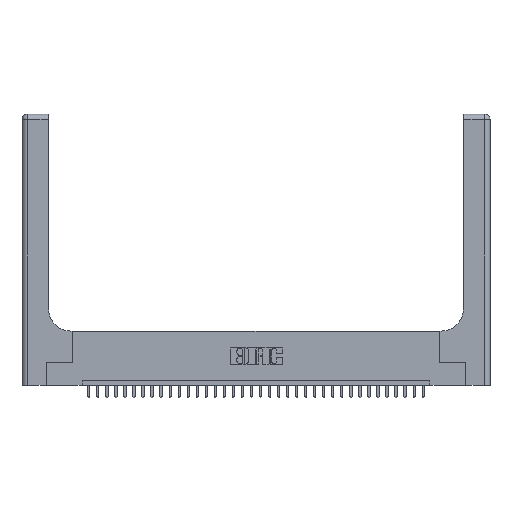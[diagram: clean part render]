
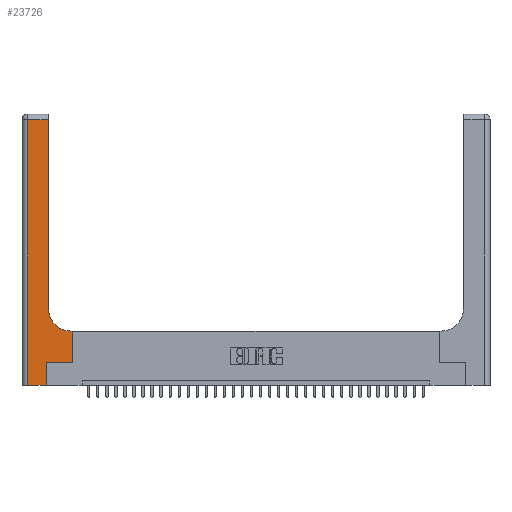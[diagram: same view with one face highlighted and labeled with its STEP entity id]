
A CAD part, top view. The second image highlights one B-rep face of the part: STEP entity #23726.
In plain terms, the highlighted planar face has unit normal (0, 0, 1).
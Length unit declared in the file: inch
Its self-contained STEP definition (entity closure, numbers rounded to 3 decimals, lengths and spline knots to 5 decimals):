
#28 = AXIS2_PLACEMENT_3D ( 'NONE', #9016, #14420, #17195 ) ;
#108 = CARTESIAN_POINT ( 'NONE',  ( 0.06, 0., 0.37 ) ) ;
#949 = VERTEX_POINT ( 'NONE', #8514 ) ;
#1142 = VERTEX_POINT ( 'NONE', #10411 ) ;
#1593 = EDGE_CURVE ( 'NONE', #949, #24150, #19657, .T. ) ;
#1617 = DIRECTION ( 'NONE',  ( 0., -1., 0. ) ) ;
#1848 = DIRECTION ( 'NONE',  ( 1., 0., 0. ) ) ;
#2084 = CARTESIAN_POINT ( 'NONE',  ( 0.269, 0.25, 0.37 ) ) ;
#3332 = CARTESIAN_POINT ( 'NONE',  ( 0.5415, 0.6, 0.37 ) ) ;
#3934 = LINE ( 'NONE', #2084, #21708 ) ;
#3965 = DIRECTION ( 'NONE',  ( -1., 0., 0. ) ) ;
#4479 = VERTEX_POINT ( 'NONE', #31100 ) ;
#5057 = DIRECTION ( 'NONE',  ( -1., 0., 0. ) ) ;
#6940 = DIRECTION ( 'NONE',  ( 0., 1., 0. ) ) ;
#7277 = EDGE_CURVE ( 'NONE', #1142, #15568, #17234, .T. ) ;
#7863 = VERTEX_POINT ( 'NONE', #3332 ) ;
#8049 = ORIENTED_EDGE ( 'NONE', *, *, #18029, .T. ) ;
#8156 = VECTOR ( 'NONE', #6940, 39.37008 ) ;
#8331 = VECTOR ( 'NONE', #9552, 39.37008 ) ;
#8478 = CARTESIAN_POINT ( 'NONE',  ( 0., 2.94, 0.37 ) ) ;
#8514 = CARTESIAN_POINT ( 'NONE',  ( 0.06, 2.94, 0.37 ) ) ;
#9016 = CARTESIAN_POINT ( 'NONE',  ( 0.5415, 0.85, 0.37 ) ) ;
#9070 = VECTOR ( 'NONE', #29698, 39.37008 ) ;
#9345 = ORIENTED_EDGE ( 'NONE', *, *, #1593, .T. ) ;
#9371 = LINE ( 'NONE', #12510, #17203 ) ;
#9552 = DIRECTION ( 'NONE',  ( 1., 0., 0. ) ) ;
#9808 = ORIENTED_EDGE ( 'NONE', *, *, #16671, .T. ) ;
#10411 = CARTESIAN_POINT ( 'NONE',  ( 0.5585, 0.25, 0.37 ) ) ;
#10804 = ORIENTED_EDGE ( 'NONE', *, *, #7277, .T. ) ;
#11607 = CARTESIAN_POINT ( 'NONE',  ( 0., 3., 0.37 ) ) ;
#11647 = LINE ( 'NONE', #25682, #8331 ) ;
#12274 = CARTESIAN_POINT ( 'NONE',  ( 0.2915, 3., 0.37 ) ) ;
#12510 = CARTESIAN_POINT ( 'NONE',  ( 0.269, 0., 0.37 ) ) ;
#12980 = CARTESIAN_POINT ( 'NONE',  ( 0.2915, 2.94, 0.37 ) ) ;
#14412 = CIRCLE ( 'NONE', #28, 0.25 ) ;
#14420 = DIRECTION ( 'NONE',  ( 0., 0., -1. ) ) ;
#14799 = EDGE_CURVE ( 'NONE', #7863, #29219, #14412, .T. ) ;
#15288 = DIRECTION ( 'NONE',  ( 0., 1., 0. ) ) ;
#15568 = VERTEX_POINT ( 'NONE', #27594 ) ;
#15746 = DIRECTION ( 'NONE',  ( 0., 1., 0. ) ) ;
#15873 = EDGE_CURVE ( 'NONE', #4479, #26837, #9371, .T. ) ;
#16080 = LINE ( 'NONE', #31485, #26107 ) ;
#16084 = LINE ( 'NONE', #8478, #9070 ) ;
#16671 = EDGE_CURVE ( 'NONE', #15568, #7863, #16080, .T. ) ;
#17195 = DIRECTION ( 'NONE',  ( 1., 0., 0. ) ) ;
#17203 = VECTOR ( 'NONE', #15288, 39.37008 ) ;
#17234 = LINE ( 'NONE', #32418, #8156 ) ;
#17813 = LINE ( 'NONE', #12274, #29883 ) ;
#18029 = EDGE_CURVE ( 'NONE', #29219, #22592, #17813, .T. ) ;
#18394 = FACE_OUTER_BOUND ( 'NONE', #28026, .T. ) ;
#18837 = VECTOR ( 'NONE', #1617, 39.37008 ) ;
#19054 = ORIENTED_EDGE ( 'NONE', *, *, #15873, .T. ) ;
#19657 = LINE ( 'NONE', #22809, #18837 ) ;
#20037 = DIRECTION ( 'NONE',  ( 0., 0., -1. ) ) ;
#21046 = ORIENTED_EDGE ( 'NONE', *, *, #23815, .T. ) ;
#21708 = VECTOR ( 'NONE', #1848, 39.37008 ) ;
#22373 = ORIENTED_EDGE ( 'NONE', *, *, #14799, .T. ) ;
#22453 = EDGE_CURVE ( 'NONE', #24150, #4479, #11647, .T. ) ;
#22592 = VERTEX_POINT ( 'NONE', #12980 ) ;
#22701 = PLANE ( 'NONE',  #33259 ) ;
#22809 = CARTESIAN_POINT ( 'NONE',  ( 0.06, 3., 0.37 ) ) ;
#23487 = ORIENTED_EDGE ( 'NONE', *, *, #22453, .T. ) ;
#23726 = ADVANCED_FACE ( 'NONE', ( #18394 ), #22701, .F. ) ;
#23815 = EDGE_CURVE ( 'NONE', #26837, #1142, #3934, .T. ) ;
#24150 = VERTEX_POINT ( 'NONE', #108 ) ;
#25627 = ORIENTED_EDGE ( 'NONE', *, *, #27071, .T. ) ;
#25682 = CARTESIAN_POINT ( 'NONE',  ( 0., 0., 0.37 ) ) ;
#26107 = VECTOR ( 'NONE', #5057, 39.37008 ) ;
#26837 = VERTEX_POINT ( 'NONE', #34325 ) ;
#27071 = EDGE_CURVE ( 'NONE', #22592, #949, #16084, .T. ) ;
#27594 = CARTESIAN_POINT ( 'NONE',  ( 0.5585, 0.6, 0.37 ) ) ;
#28026 = EDGE_LOOP ( 'NONE', ( #8049, #25627, #9345, #23487, #19054, #21046, #10804, #9808, #22373 ) ) ;
#29219 = VERTEX_POINT ( 'NONE', #29317 ) ;
#29317 = CARTESIAN_POINT ( 'NONE',  ( 0.2915, 0.85, 0.37 ) ) ;
#29698 = DIRECTION ( 'NONE',  ( -1., 0., 0. ) ) ;
#29883 = VECTOR ( 'NONE', #15746, 39.37008 ) ;
#31100 = CARTESIAN_POINT ( 'NONE',  ( 0.269, 0., 0.37 ) ) ;
#31485 = CARTESIAN_POINT ( 'NONE',  ( 0.2915, 0.6, 0.37 ) ) ;
#32418 = CARTESIAN_POINT ( 'NONE',  ( 0.5585, 0.25, 0.37 ) ) ;
#33259 = AXIS2_PLACEMENT_3D ( 'NONE', #11607, #20037, #3965 ) ;
#34325 = CARTESIAN_POINT ( 'NONE',  ( 0.269, 0.25, 0.37 ) ) ;
